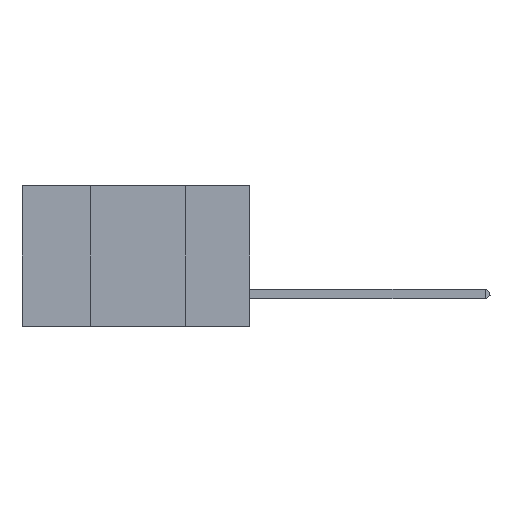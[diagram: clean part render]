
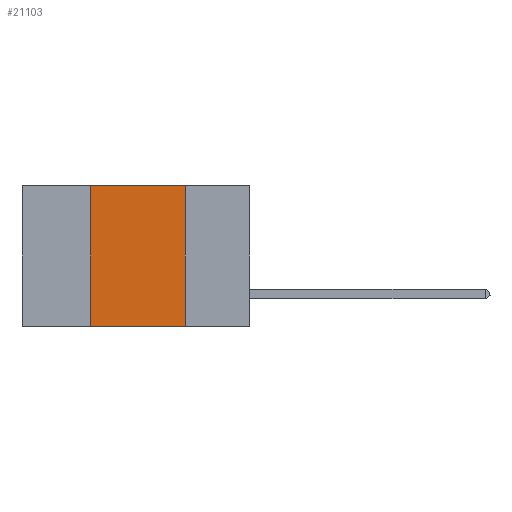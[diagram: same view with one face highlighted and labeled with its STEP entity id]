
A CAD part, left-side view. The second image highlights one B-rep face of the part: STEP entity #21103.
In plain terms, the highlighted planar face has unit normal (-1, 0, 0).
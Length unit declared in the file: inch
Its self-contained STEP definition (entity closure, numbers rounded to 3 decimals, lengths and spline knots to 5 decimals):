
#231 = CARTESIAN_POINT ( 'NONE',  ( 0., 0.42, 0. ) ) ;
#381 = DIRECTION ( 'NONE',  ( 0., 0., -1. ) ) ;
#443 = PLANE ( 'NONE',  #7063 ) ;
#1688 = VERTEX_POINT ( 'NONE', #11345 ) ;
#2114 = ORIENTED_EDGE ( 'NONE', *, *, #16999, .F. ) ;
#2934 = VERTEX_POINT ( 'NONE', #6043 ) ;
#3244 = ORIENTED_EDGE ( 'NONE', *, *, #14020, .T. ) ;
#5879 = CARTESIAN_POINT ( 'NONE',  ( 0., 0.6, 0. ) ) ;
#6043 = CARTESIAN_POINT ( 'NONE',  ( 0., 0.42, 0. ) ) ;
#6094 = LINE ( 'NONE', #6911, #7155 ) ;
#6911 = CARTESIAN_POINT ( 'NONE',  ( 0., 0.17, 0. ) ) ;
#7063 = AXIS2_PLACEMENT_3D ( 'NONE', #5879, #11013, #18093 ) ;
#7155 = VECTOR ( 'NONE', #381, 39.37008 ) ;
#7284 = VERTEX_POINT ( 'NONE', #20815 ) ;
#7495 = ORIENTED_EDGE ( 'NONE', *, *, #12420, .F. ) ;
#7646 = LINE ( 'NONE', #231, #19021 ) ;
#7960 = DIRECTION ( 'NONE',  ( 0., -1., 0. ) ) ;
#8239 = EDGE_CURVE ( 'NONE', #2934, #7284, #21127, .T. ) ;
#8418 = VERTEX_POINT ( 'NONE', #9037 ) ;
#9037 = CARTESIAN_POINT ( 'NONE',  ( 0., 0.17, -0.37 ) ) ;
#9108 = DIRECTION ( 'NONE',  ( 0., 0., 1. ) ) ;
#9520 = LINE ( 'NONE', #22313, #11456 ) ;
#11013 = DIRECTION ( 'NONE',  ( 1., 0., 0. ) ) ;
#11345 = CARTESIAN_POINT ( 'NONE',  ( 0., 0.42, -0.37 ) ) ;
#11456 = VECTOR ( 'NONE', #7960, 39.37008 ) ;
#12420 = EDGE_CURVE ( 'NONE', #1688, #2934, #7646, .T. ) ;
#14020 = EDGE_CURVE ( 'NONE', #1688, #8418, #9520, .T. ) ;
#15602 = CARTESIAN_POINT ( 'NONE',  ( 0., 0.6, 0. ) ) ;
#16260 = EDGE_LOOP ( 'NONE', ( #2114, #20401, #7495, #3244 ) ) ;
#16590 = VECTOR ( 'NONE', #22217, 39.37008 ) ;
#16999 = EDGE_CURVE ( 'NONE', #7284, #8418, #6094, .T. ) ;
#18093 = DIRECTION ( 'NONE',  ( 0., 0., -1. ) ) ;
#18133 = FACE_OUTER_BOUND ( 'NONE', #16260, .T. ) ;
#19021 = VECTOR ( 'NONE', #9108, 39.37008 ) ;
#20401 = ORIENTED_EDGE ( 'NONE', *, *, #8239, .F. ) ;
#20815 = CARTESIAN_POINT ( 'NONE',  ( 0., 0.17, 0. ) ) ;
#21103 = ADVANCED_FACE ( 'NONE', ( #18133 ), #443, .F. ) ;
#21127 = LINE ( 'NONE', #15602, #16590 ) ;
#22217 = DIRECTION ( 'NONE',  ( 0., -1., 0. ) ) ;
#22313 = CARTESIAN_POINT ( 'NONE',  ( 0., 0.6, -0.37 ) ) ;
